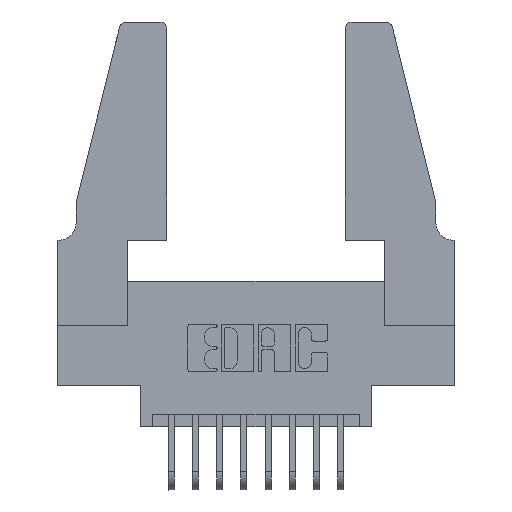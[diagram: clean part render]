
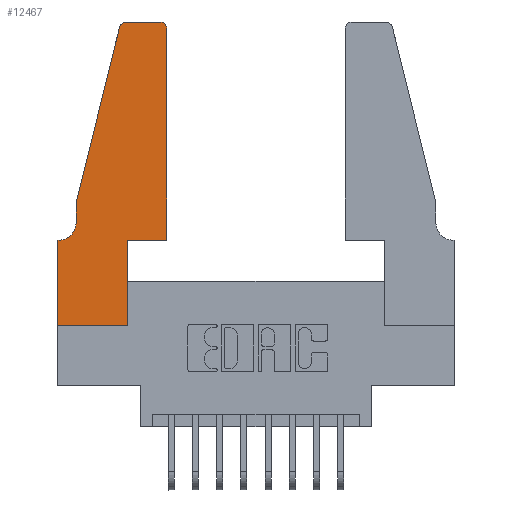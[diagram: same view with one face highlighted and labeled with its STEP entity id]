
A CAD part, top view. The second image highlights one B-rep face of the part: STEP entity #12467.
In plain terms, the highlighted planar face has unit normal (0, 0, 1).
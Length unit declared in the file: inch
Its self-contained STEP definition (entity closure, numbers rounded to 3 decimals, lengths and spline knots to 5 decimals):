
#63 = FACE_OUTER_BOUND ( 'NONE', #10046, .T. ) ;
#100 = DIRECTION ( 'NONE',  ( 1., 0., 0. ) ) ;
#221 = ORIENTED_EDGE ( 'NONE', *, *, #5731, .T. ) ;
#601 = LINE ( 'NONE', #9260, #926 ) ;
#720 = CARTESIAN_POINT ( 'NONE',  ( 0., 0., 0.37 ) ) ;
#725 = CARTESIAN_POINT ( 'NONE',  ( 0.2865, 0.35, 0.37 ) ) ;
#825 = ORIENTED_EDGE ( 'NONE', *, *, #2914, .T. ) ;
#915 = LINE ( 'NONE', #8984, #5910 ) ;
#926 = VECTOR ( 'NONE', #10259, 39.37008 ) ;
#938 = CARTESIAN_POINT ( 'NONE',  ( 0.4205, 1.22, 0.37 ) ) ;
#1324 = EDGE_CURVE ( 'NONE', #10539, #11076, #7746, .T. ) ;
#1372 = CIRCLE ( 'NONE', #1642, 0.07 ) ;
#1475 = AXIS2_PLACEMENT_3D ( 'NONE', #938, #7960, #1929 ) ;
#1528 = CARTESIAN_POINT ( 'NONE',  ( 0.284, 1.25, 0.37 ) ) ;
#1532 = CIRCLE ( 'NONE', #1475, 0.03 ) ;
#1642 = AXIS2_PLACEMENT_3D ( 'NONE', #2681, #9697, #3689 ) ;
#1892 = EDGE_CURVE ( 'NONE', #12658, #5198, #4290, .T. ) ;
#1916 = CARTESIAN_POINT ( 'NONE',  ( 0.284, 1.22, 0.37 ) ) ;
#1929 = DIRECTION ( 'NONE',  ( 1., 0., 0. ) ) ;
#1972 = VECTOR ( 'NONE', #11552, 39.37008 ) ;
#1982 = CARTESIAN_POINT ( 'NONE',  ( 0.2865, 0., 0.37 ) ) ;
#2066 = CARTESIAN_POINT ( 'NONE',  ( 0.0055, 0.35, 0.37 ) ) ;
#2072 = CARTESIAN_POINT ( 'NONE',  ( 0., 0.35, 0.37 ) ) ;
#2081 = CARTESIAN_POINT ( 'NONE',  ( 0.4505, 0.35, 0.37 ) ) ;
#2333 = CARTESIAN_POINT ( 'NONE',  ( 0.0755, 0.5, 0.37 ) ) ;
#2553 = EDGE_CURVE ( 'NONE', #6866, #4931, #9759, .T. ) ;
#2681 = CARTESIAN_POINT ( 'NONE',  ( 0.0055, 0.42, 0.37 ) ) ;
#2914 = EDGE_CURVE ( 'NONE', #11076, #6063, #6585, .T. ) ;
#2927 = DIRECTION ( 'NONE',  ( 1., 0., 0. ) ) ;
#3132 = CARTESIAN_POINT ( 'NONE',  ( 0., 0., 0.37 ) ) ;
#3332 = DIRECTION ( 'NONE',  ( 0., -1., 0. ) ) ;
#3550 = CARTESIAN_POINT ( 'NONE',  ( 0.4505, 0.35, 0.37 ) ) ;
#3689 = DIRECTION ( 'NONE',  ( -1., 0., 0. ) ) ;
#3817 = DIRECTION ( 'NONE',  ( -1., 0., 0. ) ) ;
#3871 = VECTOR ( 'NONE', #7063, 39.37008 ) ;
#4004 = CARTESIAN_POINT ( 'NONE',  ( 0.4505, 0.35, 0.37 ) ) ;
#4124 = DIRECTION ( 'NONE',  ( 0., -1., 0. ) ) ;
#4180 = LINE ( 'NONE', #2081, #3871 ) ;
#4290 = LINE ( 'NONE', #3132, #6952 ) ;
#4309 = VECTOR ( 'NONE', #5533, 39.37008 ) ;
#4361 = EDGE_CURVE ( 'NONE', #6063, #6866, #601, .T. ) ;
#4469 = ORIENTED_EDGE ( 'NONE', *, *, #6859, .T. ) ;
#4526 = CARTESIAN_POINT ( 'NONE',  ( 0., 0., 0.37 ) ) ;
#4741 = EDGE_CURVE ( 'NONE', #9894, #7325, #915, .T. ) ;
#4814 = ORIENTED_EDGE ( 'NONE', *, *, #4741, .T. ) ;
#4832 = ORIENTED_EDGE ( 'NONE', *, *, #4361, .T. ) ;
#4921 = VECTOR ( 'NONE', #3817, 39.37008 ) ;
#4931 = VERTEX_POINT ( 'NONE', #9332 ) ;
#4951 = LINE ( 'NONE', #3550, #1972 ) ;
#5086 = PLANE ( 'NONE',  #7397 ) ;
#5198 = VERTEX_POINT ( 'NONE', #720 ) ;
#5399 = VERTEX_POINT ( 'NONE', #4004 ) ;
#5533 = DIRECTION ( 'NONE',  ( 1., 0., 0. ) ) ;
#5731 = EDGE_CURVE ( 'NONE', #5399, #8926, #4951, .T. ) ;
#5910 = VECTOR ( 'NONE', #8123, 39.37008 ) ;
#6015 = VERTEX_POINT ( 'NONE', #2066 ) ;
#6063 = VERTEX_POINT ( 'NONE', #7138 ) ;
#6089 = DIRECTION ( 'NONE',  ( 0., 0., 1. ) ) ;
#6146 = ORIENTED_EDGE ( 'NONE', *, *, #1324, .T. ) ;
#6425 = CARTESIAN_POINT ( 'NONE',  ( 0.4505, 1.22, 0.37 ) ) ;
#6585 = CIRCLE ( 'NONE', #8024, 0.03 ) ;
#6859 = EDGE_CURVE ( 'NONE', #5198, #9894, #6973, .T. ) ;
#6866 = VERTEX_POINT ( 'NONE', #10571 ) ;
#6952 = VECTOR ( 'NONE', #4124, 39.37008 ) ;
#6973 = LINE ( 'NONE', #4526, #4309 ) ;
#7063 = DIRECTION ( 'NONE',  ( 1., 0., 0. ) ) ;
#7138 = CARTESIAN_POINT ( 'NONE',  ( 0.25487, 1.22718, 0.37 ) ) ;
#7325 = VERTEX_POINT ( 'NONE', #725 ) ;
#7397 = AXIS2_PLACEMENT_3D ( 'NONE', #2072, #6089, #100 ) ;
#7421 = VECTOR ( 'NONE', #12292, 39.37008 ) ;
#7581 = LINE ( 'NONE', #7823, #4921 ) ;
#7746 = LINE ( 'NONE', #9399, #7421 ) ;
#7823 = CARTESIAN_POINT ( 'NONE',  ( 0.0755, 0.35, 0.37 ) ) ;
#7960 = DIRECTION ( 'NONE',  ( 0., 0., 1. ) ) ;
#8024 = AXIS2_PLACEMENT_3D ( 'NONE', #1916, #8947, #2927 ) ;
#8123 = DIRECTION ( 'NONE',  ( 0., 1., 0. ) ) ;
#8324 = ORIENTED_EDGE ( 'NONE', *, *, #10803, .T. ) ;
#8653 = CARTESIAN_POINT ( 'NONE',  ( 0.4205, 1.25, 0.37 ) ) ;
#8926 = VERTEX_POINT ( 'NONE', #6425 ) ;
#8947 = DIRECTION ( 'NONE',  ( 0., 0., 1. ) ) ;
#8984 = CARTESIAN_POINT ( 'NONE',  ( 0.2865, 0.35, 0.37 ) ) ;
#9260 = CARTESIAN_POINT ( 'NONE',  ( 0.0755, 0.5, 0.37 ) ) ;
#9332 = CARTESIAN_POINT ( 'NONE',  ( 0.0755, 0.42, 0.37 ) ) ;
#9399 = CARTESIAN_POINT ( 'NONE',  ( 0.2605, 1.25, 0.37 ) ) ;
#9697 = DIRECTION ( 'NONE',  ( 0., 0., -1. ) ) ;
#9759 = LINE ( 'NONE', #2333, #12131 ) ;
#9876 = EDGE_CURVE ( 'NONE', #8926, #10539, #1532, .T. ) ;
#9894 = VERTEX_POINT ( 'NONE', #1982 ) ;
#10046 = EDGE_LOOP ( 'NONE', ( #6146, #825, #4832, #12918, #10897, #11592, #11241, #4469, #4814, #8324, #221, #10196 ) ) ;
#10196 = ORIENTED_EDGE ( 'NONE', *, *, #9876, .T. ) ;
#10259 = DIRECTION ( 'NONE',  ( -0.239, -0.971, 0. ) ) ;
#10539 = VERTEX_POINT ( 'NONE', #8653 ) ;
#10540 = EDGE_CURVE ( 'NONE', #4931, #6015, #1372, .T. ) ;
#10571 = CARTESIAN_POINT ( 'NONE',  ( 0.0755, 0.5, 0.37 ) ) ;
#10803 = EDGE_CURVE ( 'NONE', #7325, #5399, #4180, .T. ) ;
#10897 = ORIENTED_EDGE ( 'NONE', *, *, #10540, .T. ) ;
#11076 = VERTEX_POINT ( 'NONE', #1528 ) ;
#11241 = ORIENTED_EDGE ( 'NONE', *, *, #1892, .T. ) ;
#11383 = CARTESIAN_POINT ( 'NONE',  ( 0., 0.35, 0.37 ) ) ;
#11552 = DIRECTION ( 'NONE',  ( 0., 1., 0. ) ) ;
#11592 = ORIENTED_EDGE ( 'NONE', *, *, #12253, .T. ) ;
#12131 = VECTOR ( 'NONE', #3332, 39.37008 ) ;
#12253 = EDGE_CURVE ( 'NONE', #6015, #12658, #7581, .T. ) ;
#12292 = DIRECTION ( 'NONE',  ( -1., 0., 0. ) ) ;
#12467 = ADVANCED_FACE ( 'NONE', ( #63 ), #5086, .T. ) ;
#12658 = VERTEX_POINT ( 'NONE', #11383 ) ;
#12918 = ORIENTED_EDGE ( 'NONE', *, *, #2553, .T. ) ;
